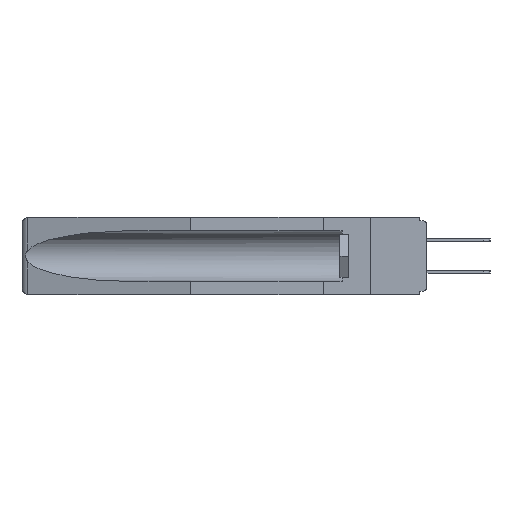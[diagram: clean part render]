
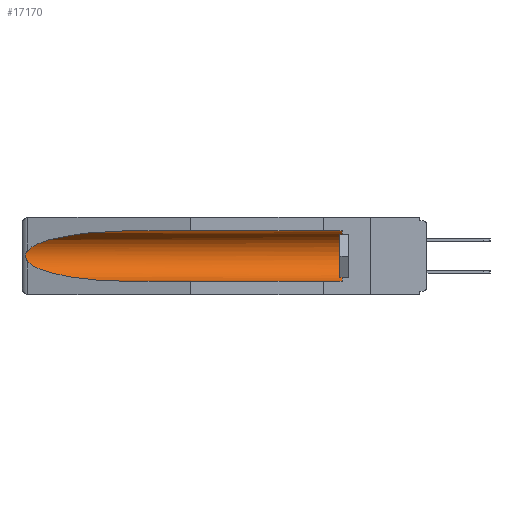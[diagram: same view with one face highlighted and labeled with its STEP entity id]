
A CAD part, left-side view. The second image highlights one B-rep face of the part: STEP entity #17170.
In plain terms, the highlighted cylindrical face has radius 2.857 mm (diameter 5.715 mm), a partial arc.
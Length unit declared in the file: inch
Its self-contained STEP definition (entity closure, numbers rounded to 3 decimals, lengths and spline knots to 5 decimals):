
#92 = EDGE_LOOP ( 'NONE', ( #7145, #12562, #24128, #14493, #16795, #1233 ) ) ;
#339 = CARTESIAN_POINT ( 'NONE',  ( 0.26537, 1.52718, -0.19328 ) ) ;
#353 = CARTESIAN_POINT ( 'NONE',  ( 0.155, -0.30754, -0.059 ) ) ;
#549 = AXIS2_PLACEMENT_3D ( 'NONE', #6473, #27549, #23113 ) ;
#773 = VERTEX_POINT ( 'NONE', #13498 ) ;
#806 = VERTEX_POINT ( 'NONE', #11350 ) ;
#1233 = ORIENTED_EDGE ( 'NONE', *, *, #18837, .T. ) ;
#3084 = EDGE_CURVE ( 'NONE', #806, #29006, #15180, .T. ) ;
#4127 =( BOUNDED_CURVE ( )  B_SPLINE_CURVE ( 3, ( #9915, #9517, #18915, #26041 ),
 .UNSPECIFIED., .F., .F. ) 
 B_SPLINE_CURVE_WITH_KNOTS ( ( 4, 4 ),
 ( 0.1948, 1.5708 ),
 .UNSPECIFIED. ) 
 CURVE ( )  GEOMETRIC_REPRESENTATION_ITEM ( )  RATIONAL_B_SPLINE_CURVE ( ( 1., 0.848, 0.848, 1. ) ) 
 REPRESENTATION_ITEM ( '' )  );
#5024 = CARTESIAN_POINT ( 'NONE',  ( 0.2675, 1.53308, -0.17534 ) ) ;
#5100 = CARTESIAN_POINT ( 'NONE',  ( 0.155, -0.30754, -0.1715 ) ) ;
#6473 = CARTESIAN_POINT ( 'NONE',  ( 0.155, 0.126, -0.1715 ) ) ;
#6976 = CARTESIAN_POINT ( 'NONE',  ( 0.21114, 1.30732, -0.059 ) ) ;
#7029 = CARTESIAN_POINT ( 'NONE',  ( 0.2673, 1.5327, -0.16383 ) ) ;
#7145 = ORIENTED_EDGE ( 'NONE', *, *, #25889, .T. ) ;
#7344 = CARTESIAN_POINT ( 'NONE',  ( 0.26597, 1.5296, -0.19026 ) ) ;
#9339 = EDGE_CURVE ( 'NONE', #25751, #22701, #27068, .T. ) ;
#9433 = CARTESIAN_POINT ( 'NONE',  ( 0.26654, 1.53092, -0.15636 ) ) ;
#9517 = CARTESIAN_POINT ( 'NONE',  ( 0.25451, 1.48313, -0.24835 ) ) ;
#9859 = DIRECTION ( 'NONE',  ( 0., 1., 0. ) ) ;
#9915 = CARTESIAN_POINT ( 'NONE',  ( 0.26537, 1.52718, -0.19328 ) ) ;
#10497 = CARTESIAN_POINT ( 'NONE',  ( 0.155, 1.07973, -0.284 ) ) ;
#11140 = CYLINDRICAL_SURFACE ( 'NONE', #18076, 0.1125 ) ;
#11267 = VERTEX_POINT ( 'NONE', #15020 ) ;
#11350 = CARTESIAN_POINT ( 'NONE',  ( 0.155, 0.126, -0.284 ) ) ;
#12562 = ORIENTED_EDGE ( 'NONE', *, *, #9339, .T. ) ;
#13498 = CARTESIAN_POINT ( 'NONE',  ( 0.155, 1.07973, -0.059 ) ) ;
#14493 = ORIENTED_EDGE ( 'NONE', *, *, #3084, .F. ) ;
#14590 = CARTESIAN_POINT ( 'NONE',  ( 0.26655, 1.53094, -0.18657 ) ) ;
#15020 = CARTESIAN_POINT ( 'NONE',  ( 0.155, 0.126, -0.059 ) ) ;
#15180 = LINE ( 'NONE', #22729, #19633 ) ;
#15840 = EDGE_CURVE ( 'NONE', #806, #11267, #17522, .T. ) ;
#15948 = FACE_OUTER_BOUND ( 'NONE', #92, .T. ) ;
#16795 = ORIENTED_EDGE ( 'NONE', *, *, #15840, .T. ) ;
#17170 = ADVANCED_FACE ( 'NONE', ( #15948 ), #11140, .F. ) ;
#17522 = CIRCLE ( 'NONE', #549, 0.1125 ) ;
#18076 = AXIS2_PLACEMENT_3D ( 'NONE', #5100, #19309, #26420 ) ;
#18581 = CARTESIAN_POINT ( 'NONE',  ( 0.25451, 1.48313, -0.09465 ) ) ;
#18837 = EDGE_CURVE ( 'NONE', #11267, #773, #25223, .T. ) ;
#18915 = CARTESIAN_POINT ( 'NONE',  ( 0.21114, 1.30732, -0.284 ) ) ;
#18961 = VECTOR ( 'NONE', #9859, 39.37008 ) ;
#19233 = CARTESIAN_POINT ( 'NONE',  ( 0.2675, 1.53308, -0.16763 ) ) ;
#19309 = DIRECTION ( 'NONE',  ( 0., 1., 0. ) ) ;
#19633 = VECTOR ( 'NONE', #24915, 39.37008 ) ;
#21137 = CARTESIAN_POINT ( 'NONE',  ( 0.155, 1.07973, -0.059 ) ) ;
#21600 =( BOUNDED_CURVE ( )  B_SPLINE_CURVE ( 3, ( #21137, #6976, #18581, #25700 ),
 .UNSPECIFIED., .F., .T. ) 
 B_SPLINE_CURVE_WITH_KNOTS ( ( 4, 4 ),
 ( 4.71239, 6.08839 ),
 .UNSPECIFIED. ) 
 CURVE ( )  GEOMETRIC_REPRESENTATION_ITEM ( )  RATIONAL_B_SPLINE_CURVE ( ( 1., 0.848, 0.848, 1. ) ) 
 REPRESENTATION_ITEM ( '' )  );
#22701 = VERTEX_POINT ( 'NONE', #30271 ) ;
#22729 = CARTESIAN_POINT ( 'NONE',  ( 0.155, -0.30754, -0.284 ) ) ;
#23113 = DIRECTION ( 'NONE',  ( 0., 0., 1. ) ) ;
#23774 = CARTESIAN_POINT ( 'NONE',  ( 0.2673, 1.53269, -0.17917 ) ) ;
#24128 = ORIENTED_EDGE ( 'NONE', *, *, #25383, .T. ) ;
#24915 = DIRECTION ( 'NONE',  ( 0., 1., 0. ) ) ;
#25223 = LINE ( 'NONE', #353, #18961 ) ;
#25383 = EDGE_CURVE ( 'NONE', #22701, #29006, #4127, .T. ) ;
#25700 = CARTESIAN_POINT ( 'NONE',  ( 0.26537, 1.52718, -0.14972 ) ) ;
#25751 = VERTEX_POINT ( 'NONE', #27527 ) ;
#25889 = EDGE_CURVE ( 'NONE', #773, #25751, #21600, .T. ) ;
#26041 = CARTESIAN_POINT ( 'NONE',  ( 0.155, 1.07973, -0.284 ) ) ;
#26420 = DIRECTION ( 'NONE',  ( 0., 0., 1. ) ) ;
#27068 = B_SPLINE_CURVE_WITH_KNOTS ( 'NONE', 3,
 ( #28496, #28691, #9433, #7029, #19233, #5024, #23774, #14590, #7344, #339 ),
 .UNSPECIFIED., .F., .F.,
 ( 4, 2, 2, 2, 4 ),
 ( 0., 0.00029, 0.00058, 0.00087, 0.00117 ),
 .UNSPECIFIED. ) ;
#27527 = CARTESIAN_POINT ( 'NONE',  ( 0.26537, 1.52718, -0.14972 ) ) ;
#27549 = DIRECTION ( 'NONE',  ( 0., -1., 0. ) ) ;
#28496 = CARTESIAN_POINT ( 'NONE',  ( 0.26537, 1.52718, -0.14972 ) ) ;
#28691 = CARTESIAN_POINT ( 'NONE',  ( 0.26597, 1.52961, -0.15275 ) ) ;
#29006 = VERTEX_POINT ( 'NONE', #10497 ) ;
#30271 = CARTESIAN_POINT ( 'NONE',  ( 0.26537, 1.52718, -0.19328 ) ) ;
